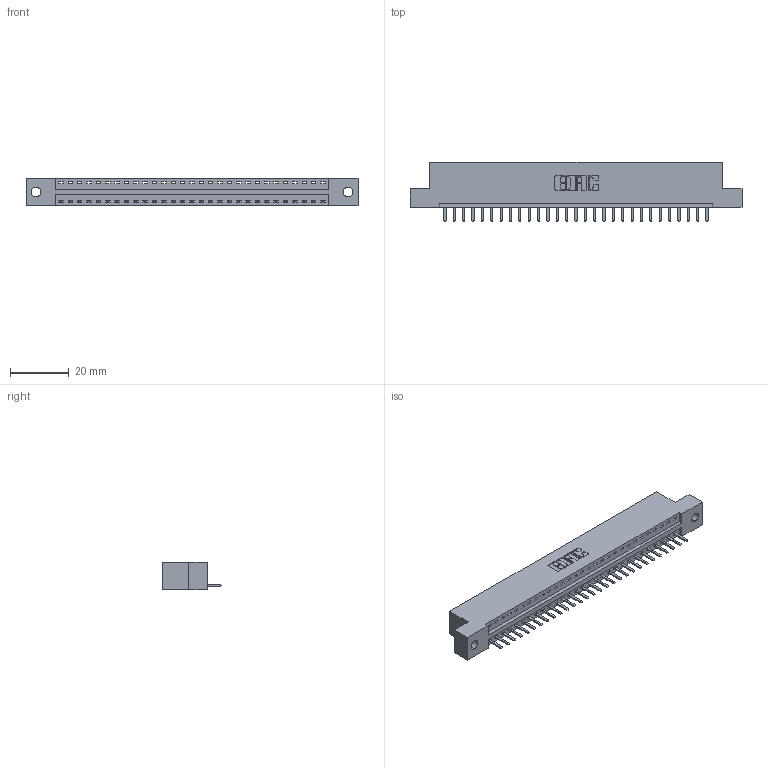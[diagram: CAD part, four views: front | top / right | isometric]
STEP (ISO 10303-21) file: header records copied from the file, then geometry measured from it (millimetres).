
FILE_DESCRIPTION (( 'STEP AP203' ), '1' );
FILE_NAME ('346-029-520-102.STEP', '2022-05-06T08:21:08', ( '' ), ( '' ), 'SwSTEP 2.0', 'SolidWorks 2020', '' );
FILE_SCHEMA (( 'CONFIG_CONTROL_DESIGN' ));
Length unit declared in the file: inch
Products named in the file (3): 345-292-001_345-293-120; 346-029-520-102; 346 Part_Flush Mounting Lugs - 0.128 Dia
Assembly tree (30 placements, depth 2):
  346-029-520-102
    346 Part_Flush Mounting Lugs - 0.128 Dia
    345-292-001_345-293-120  x29
Bounding box: 112.65 x 20.02 x 9.4 mm (x, y, z)
Volume: 10573.3 mm3; surface area: 12525.3 mm2
Topology: 30 solids, 30 shells, 1920 faces, 5665 edges, 3698 vertices
Faces by surface type: plane 1294, cylinder 626
Entity records: 19865 total; most frequent: CARTESIAN_POINT 3427, ORIENTED_EDGE 3378, DIRECTION 3027, EDGE_CURVE 1689, LINE 1437, VECTOR 1437, VERTEX_POINT 1122, AXIS2_PLACEMENT_3D 795
